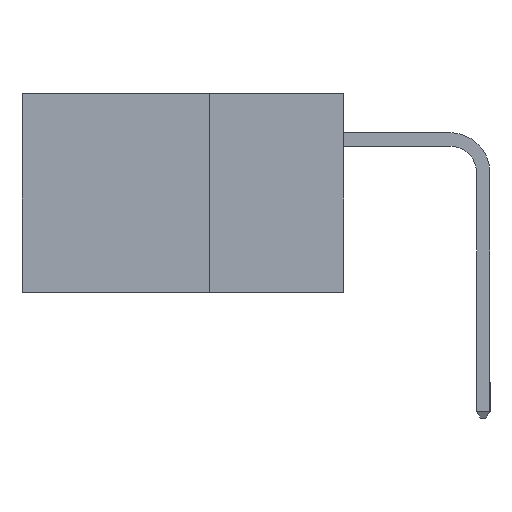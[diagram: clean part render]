
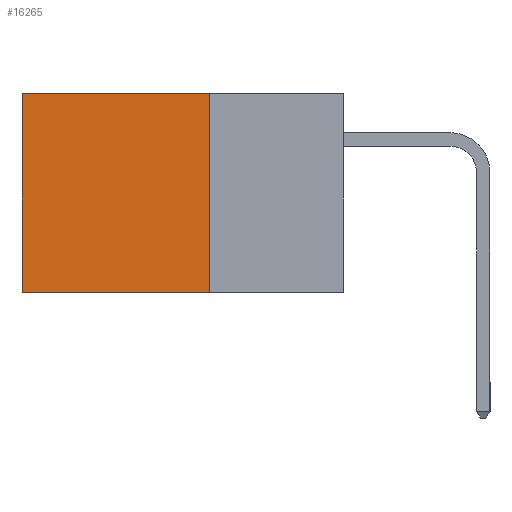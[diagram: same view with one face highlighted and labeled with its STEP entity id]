
A CAD part, left-side view. The second image highlights one B-rep face of the part: STEP entity #16265.
In plain terms, the highlighted planar face has unit normal (-1, 0, 0).
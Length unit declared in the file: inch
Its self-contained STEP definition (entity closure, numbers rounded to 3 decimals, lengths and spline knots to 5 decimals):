
#37 = CARTESIAN_POINT ( 'NONE',  ( 0.298, 0.6, 0. ) ) ;
#52 = ORIENTED_EDGE ( 'NONE', *, *, #4449, .F. ) ;
#323 = ORIENTED_EDGE ( 'NONE', *, *, #15320, .T. ) ;
#892 = DIRECTION ( 'NONE',  ( 0., 0., -1. ) ) ;
#946 = DIRECTION ( 'NONE',  ( 0., 1., 0. ) ) ;
#947 = DIRECTION ( 'NONE',  ( 0., 0., -1. ) ) ;
#1747 = FACE_OUTER_BOUND ( 'NONE', #5757, .T. ) ;
#2148 = CARTESIAN_POINT ( 'NONE',  ( 0.298, 0.25, 0. ) ) ;
#2399 = CARTESIAN_POINT ( 'NONE',  ( 0.298, 0.25, -0.37 ) ) ;
#3684 = VECTOR ( 'NONE', #947, 39.37008 ) ;
#3795 = DIRECTION ( 'NONE',  ( 0., 1., 0. ) ) ;
#3839 = VECTOR ( 'NONE', #4456, 39.37008 ) ;
#3978 = EDGE_CURVE ( 'NONE', #9968, #9883, #7303, .T. ) ;
#4255 = VECTOR ( 'NONE', #3795, 39.37008 ) ;
#4449 = EDGE_CURVE ( 'NONE', #10731, #9968, #10716, .T. ) ;
#4456 = DIRECTION ( 'NONE',  ( 0., 0., -1. ) ) ;
#4841 = VERTEX_POINT ( 'NONE', #37 ) ;
#5125 = CARTESIAN_POINT ( 'NONE',  ( 0.298, 0.6, -0.37 ) ) ;
#5757 = EDGE_LOOP ( 'NONE', ( #10822, #11076, #52, #323 ) ) ;
#7303 = LINE ( 'NONE', #9801, #4255 ) ;
#8612 = DIRECTION ( 'NONE',  ( 1., 0., 0. ) ) ;
#9801 = CARTESIAN_POINT ( 'NONE',  ( 0.298, 0.25, -0.37 ) ) ;
#9883 = VERTEX_POINT ( 'NONE', #5125 ) ;
#9968 = VERTEX_POINT ( 'NONE', #2399 ) ;
#10497 = EDGE_CURVE ( 'NONE', #4841, #9883, #10967, .T. ) ;
#10716 = LINE ( 'NONE', #12009, #3839 ) ;
#10731 = VERTEX_POINT ( 'NONE', #12971 ) ;
#10822 = ORIENTED_EDGE ( 'NONE', *, *, #10497, .T. ) ;
#10967 = LINE ( 'NONE', #16246, #3684 ) ;
#11076 = ORIENTED_EDGE ( 'NONE', *, *, #3978, .F. ) ;
#12009 = CARTESIAN_POINT ( 'NONE',  ( 0.298, 0.25, 0. ) ) ;
#12682 = LINE ( 'NONE', #15015, #16386 ) ;
#12971 = CARTESIAN_POINT ( 'NONE',  ( 0.298, 0.25, 0. ) ) ;
#15015 = CARTESIAN_POINT ( 'NONE',  ( 0.298, 0.25, 0. ) ) ;
#15320 = EDGE_CURVE ( 'NONE', #10731, #4841, #12682, .T. ) ;
#16187 = PLANE ( 'NONE',  #16260 ) ;
#16246 = CARTESIAN_POINT ( 'NONE',  ( 0.298, 0.6, 0. ) ) ;
#16260 = AXIS2_PLACEMENT_3D ( 'NONE', #2148, #8612, #892 ) ;
#16265 = ADVANCED_FACE ( 'NONE', ( #1747 ), #16187, .F. ) ;
#16386 = VECTOR ( 'NONE', #946, 39.37008 ) ;
